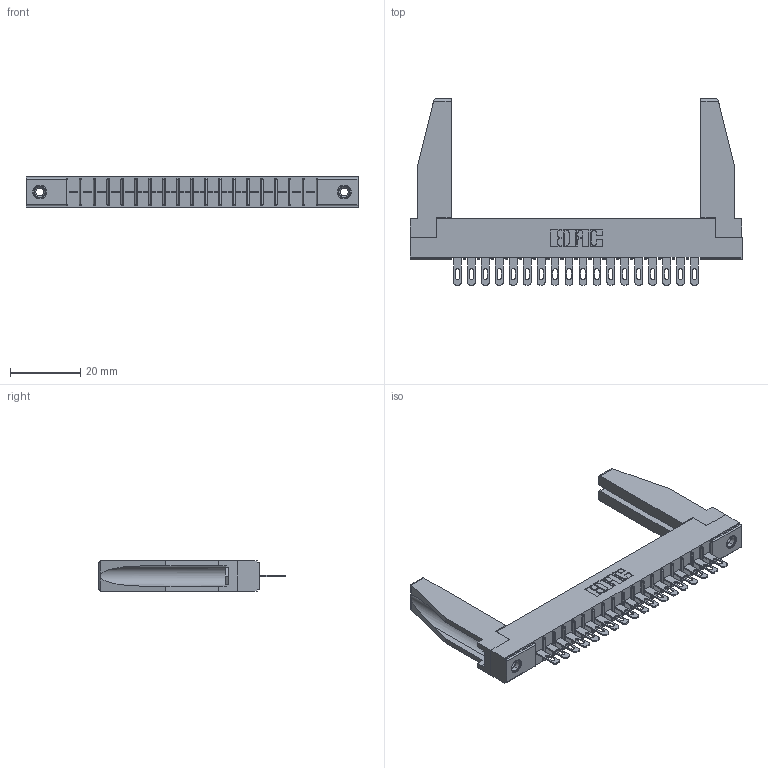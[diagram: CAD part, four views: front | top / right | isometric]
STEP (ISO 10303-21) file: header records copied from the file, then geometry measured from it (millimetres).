
FILE_DESCRIPTION (( 'STEP AP203' ), '1' );
FILE_NAME ('356-018-400-178.STEP', '2020-09-23T13:25:24', ( '' ), ( '' ), 'SwSTEP 2.0', 'SolidWorks 2020', '' );
FILE_SCHEMA (( 'CONFIG_CONTROL_DESIGN' ));
Length unit declared in the file: inch
Products named in the file (5): 307-220-078; 306 Part_.156 Dia; 345-250-001_345-250-001-102; 306-290-001_100; 356-018-400-178
Assembly tree (23 placements, depth 2):
  356-018-400-178
    306 Part_.156 Dia
    306-290-001_100  x18
    345-250-001_345-250-001-102  x2
    307-220-078  x2
Bounding box: 94.34 x 52.91 x 8.71 mm (x, y, z)
Volume: 10481.4 mm3; surface area: 13591.4 mm2
Topology: 23 solids, 23 shells, 1614 faces, 4516 edges, 2904 vertices
Faces by surface type: plane 1052, cylinder 474, sphere 72, cone 12, torus 4
Entity records: 22498 total; most frequent: CARTESIAN_POINT 3775, ORIENTED_EDGE 3698, DIRECTION 3677, EDGE_CURVE 1849, VECTOR 1433, LINE 1433, VERTEX_POINT 1178, AXIS2_PLACEMENT_3D 1122
